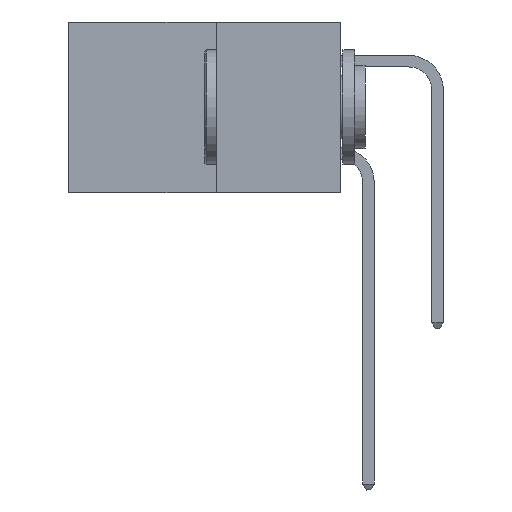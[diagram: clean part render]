
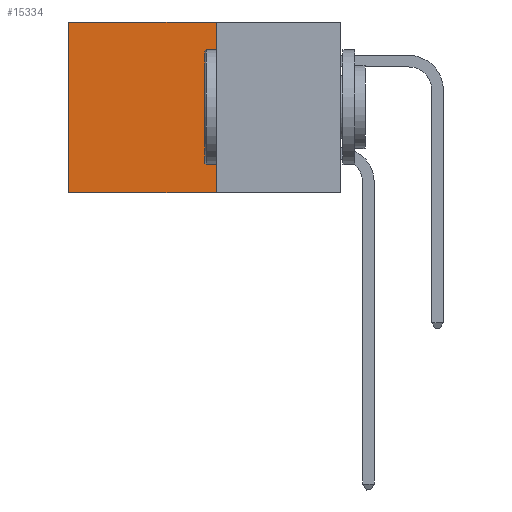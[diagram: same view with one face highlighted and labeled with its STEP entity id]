
A CAD part, left-side view. The second image highlights one B-rep face of the part: STEP entity #15334.
In plain terms, the highlighted planar face has unit normal (-1, 0, 0).
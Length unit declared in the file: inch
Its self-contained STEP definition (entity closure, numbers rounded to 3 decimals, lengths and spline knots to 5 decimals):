
#397 = ORIENTED_EDGE ( 'NONE', *, *, #11469, .F. ) ;
#1295 = CARTESIAN_POINT ( 'NONE',  ( 0.277, 0.27, -0.37 ) ) ;
#1897 = EDGE_LOOP ( 'NONE', ( #5195, #17503, #397, #6681 ) ) ;
#3615 = DIRECTION ( 'NONE',  ( 1., 0., 0. ) ) ;
#4017 = VECTOR ( 'NONE', #17220, 39.37008 ) ;
#5195 = ORIENTED_EDGE ( 'NONE', *, *, #10740, .T. ) ;
#6570 = VECTOR ( 'NONE', #17575, 39.37008 ) ;
#6681 = ORIENTED_EDGE ( 'NONE', *, *, #7201, .T. ) ;
#6869 = CARTESIAN_POINT ( 'NONE',  ( 0.277, 0.59, 0. ) ) ;
#7201 = EDGE_CURVE ( 'NONE', #22135, #19397, #10235, .T. ) ;
#7995 = FACE_OUTER_BOUND ( 'NONE', #1897, .T. ) ;
#10235 = LINE ( 'NONE', #25984, #4017 ) ;
#10720 = EDGE_CURVE ( 'NONE', #24910, #24283, #12057, .T. ) ;
#10740 = EDGE_CURVE ( 'NONE', #19397, #24283, #28871, .T. ) ;
#11420 = DIRECTION ( 'NONE',  ( 0., 0., -1. ) ) ;
#11469 = EDGE_CURVE ( 'NONE', #22135, #24910, #18076, .T. ) ;
#12057 = LINE ( 'NONE', #1295, #6570 ) ;
#12944 = PLANE ( 'NONE',  #20235 ) ;
#13431 = VECTOR ( 'NONE', #11420, 39.37008 ) ;
#14499 = CARTESIAN_POINT ( 'NONE',  ( 0.277, 0.27, -0.37 ) ) ;
#15037 = CARTESIAN_POINT ( 'NONE',  ( 0.277, 0.27, -0.37 ) ) ;
#15298 = CARTESIAN_POINT ( 'NONE',  ( 0.277, 0.59, -0.37 ) ) ;
#15334 = ADVANCED_FACE ( 'NONE', ( #7995 ), #12944, .F. ) ;
#16902 = CARTESIAN_POINT ( 'NONE',  ( 0.277, 0.27, 0. ) ) ;
#17220 = DIRECTION ( 'NONE',  ( 0., 1., 0. ) ) ;
#17503 = ORIENTED_EDGE ( 'NONE', *, *, #10720, .F. ) ;
#17575 = DIRECTION ( 'NONE',  ( 0., 1., 0. ) ) ;
#18076 = LINE ( 'NONE', #25185, #13431 ) ;
#19397 = VERTEX_POINT ( 'NONE', #6869 ) ;
#19829 = DIRECTION ( 'NONE',  ( 0., 0., -1. ) ) ;
#20235 = AXIS2_PLACEMENT_3D ( 'NONE', #15037, #3615, #19829 ) ;
#22135 = VERTEX_POINT ( 'NONE', #16902 ) ;
#22841 = VECTOR ( 'NONE', #24539, 39.37008 ) ;
#24083 = CARTESIAN_POINT ( 'NONE',  ( 0.277, 0.59, -0.37 ) ) ;
#24283 = VERTEX_POINT ( 'NONE', #24083 ) ;
#24539 = DIRECTION ( 'NONE',  ( 0., 0., -1. ) ) ;
#24910 = VERTEX_POINT ( 'NONE', #14499 ) ;
#25185 = CARTESIAN_POINT ( 'NONE',  ( 0.277, 0.27, -0.37 ) ) ;
#25984 = CARTESIAN_POINT ( 'NONE',  ( 0.277, 0.27, 0. ) ) ;
#28871 = LINE ( 'NONE', #15298, #22841 ) ;
